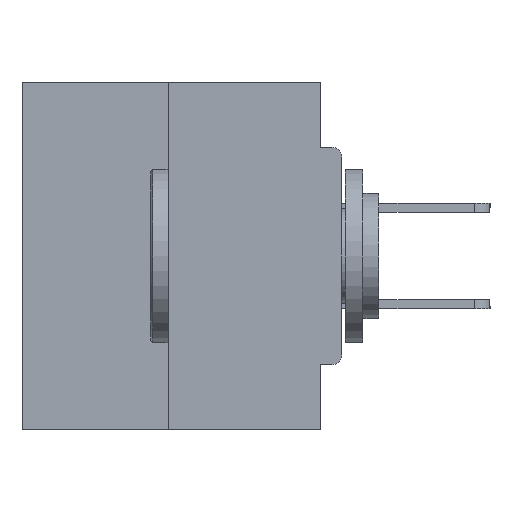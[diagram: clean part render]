
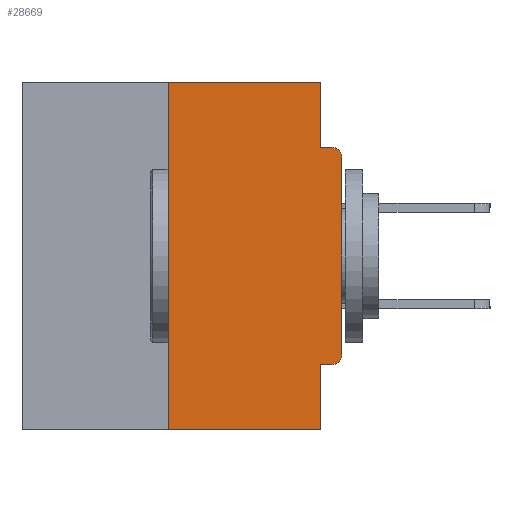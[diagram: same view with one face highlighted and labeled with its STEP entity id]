
A CAD part, left-side view. The second image highlights one B-rep face of the part: STEP entity #28669.
In plain terms, the highlighted planar face has unit normal (-1, 0, 0).
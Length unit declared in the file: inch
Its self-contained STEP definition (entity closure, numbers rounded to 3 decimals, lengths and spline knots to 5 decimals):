
#170 = AXIS2_PLACEMENT_3D ( 'NONE', #29297, #12699, #24218 ) ;
#797 = CIRCLE ( 'NONE', #20504, 0.015 ) ;
#966 = CARTESIAN_POINT ( 'NONE',  ( 0., 0.46, 0. ) ) ;
#1132 = VERTEX_POINT ( 'NONE', #33393 ) ;
#2004 = VERTEX_POINT ( 'NONE', #34199 ) ;
#2018 = CARTESIAN_POINT ( 'NONE',  ( 0., 0., 0. ) ) ;
#2049 = CARTESIAN_POINT ( 'NONE',  ( 0., 0.015, -0.0935 ) ) ;
#2283 = VECTOR ( 'NONE', #7430, 39.37008 ) ;
#2416 = DIRECTION ( 'NONE',  ( 0., 0., -1. ) ) ;
#3641 = ORIENTED_EDGE ( 'NONE', *, *, #21033, .T. ) ;
#3887 = ORIENTED_EDGE ( 'NONE', *, *, #13370, .F. ) ;
#4322 = CARTESIAN_POINT ( 'NONE',  ( 0., 0., -0.0935 ) ) ;
#4519 = CARTESIAN_POINT ( 'NONE',  ( 0., 0.25, -0.5 ) ) ;
#6406 = CARTESIAN_POINT ( 'NONE',  ( 0., 0.25, 0. ) ) ;
#6606 = LINE ( 'NONE', #4322, #2283 ) ;
#7320 = ORIENTED_EDGE ( 'NONE', *, *, #13843, .F. ) ;
#7430 = DIRECTION ( 'NONE',  ( 0., -1., 0. ) ) ;
#7748 = VERTEX_POINT ( 'NONE', #35030 ) ;
#8497 = EDGE_CURVE ( 'NONE', #1132, #11065, #6606, .T. ) ;
#8674 = ORIENTED_EDGE ( 'NONE', *, *, #22749, .T. ) ;
#8879 = VECTOR ( 'NONE', #33861, 39.37008 ) ;
#9446 = VECTOR ( 'NONE', #20384, 39.37008 ) ;
#9640 = CARTESIAN_POINT ( 'NONE',  ( 0., 0., -0.1085 ) ) ;
#9880 = EDGE_CURVE ( 'NONE', #20955, #14867, #30779, .T. ) ;
#10159 = CARTESIAN_POINT ( 'NONE',  ( 0., 0.015, -0.3915 ) ) ;
#10574 = CARTESIAN_POINT ( 'NONE',  ( 0., 0.015, -0.4065 ) ) ;
#10681 = CARTESIAN_POINT ( 'NONE',  ( 0., 0.46, -0.5 ) ) ;
#11065 = VERTEX_POINT ( 'NONE', #2049 ) ;
#12275 = EDGE_CURVE ( 'NONE', #13109, #32064, #32532, .T. ) ;
#12554 = LINE ( 'NONE', #6406, #8879 ) ;
#12572 = PLANE ( 'NONE',  #170 ) ;
#12699 = DIRECTION ( 'NONE',  ( 1., 0., 0. ) ) ;
#12783 = AXIS2_PLACEMENT_3D ( 'NONE', #21196, #20721, #34601 ) ;
#12846 = DIRECTION ( 'NONE',  ( -1., 0., 0. ) ) ;
#13091 = LINE ( 'NONE', #2018, #30837 ) ;
#13109 = VERTEX_POINT ( 'NONE', #4519 ) ;
#13370 = EDGE_CURVE ( 'NONE', #13109, #7748, #12554, .T. ) ;
#13621 = EDGE_CURVE ( 'NONE', #17387, #1132, #32442, .T. ) ;
#13722 = CARTESIAN_POINT ( 'NONE',  ( 0., 0.031, 0. ) ) ;
#13843 = EDGE_CURVE ( 'NONE', #7748, #17387, #17719, .T. ) ;
#14002 = EDGE_CURVE ( 'NONE', #20955, #2004, #797, .T. ) ;
#14108 = CARTESIAN_POINT ( 'NONE',  ( 0., 0.031, -0.5 ) ) ;
#14200 = EDGE_CURVE ( 'NONE', #14867, #32064, #22891, .T. ) ;
#14867 = VERTEX_POINT ( 'NONE', #21730 ) ;
#14953 = CARTESIAN_POINT ( 'NONE',  ( 0., 0.031, 0. ) ) ;
#16198 = FACE_OUTER_BOUND ( 'NONE', #16829, .T. ) ;
#16272 = DIRECTION ( 'NONE',  ( 0., -1., 0. ) ) ;
#16620 = DIRECTION ( 'NONE',  ( 0., 0., -1. ) ) ;
#16829 = EDGE_LOOP ( 'NONE', ( #7320, #3887, #19017, #27367, #26257, #17218, #3641, #8674, #25823, #29649 ) ) ;
#17218 = ORIENTED_EDGE ( 'NONE', *, *, #14002, .T. ) ;
#17387 = VERTEX_POINT ( 'NONE', #14953 ) ;
#17719 = LINE ( 'NONE', #966, #9446 ) ;
#17740 = CARTESIAN_POINT ( 'NONE',  ( 0., 0., -0.4065 ) ) ;
#18272 = VECTOR ( 'NONE', #16272, 39.37008 ) ;
#19017 = ORIENTED_EDGE ( 'NONE', *, *, #12275, .T. ) ;
#19019 = CARTESIAN_POINT ( 'NONE',  ( 0., 0.031, -0.5 ) ) ;
#20384 = DIRECTION ( 'NONE',  ( 0., -1., 0. ) ) ;
#20504 = AXIS2_PLACEMENT_3D ( 'NONE', #10159, #12846, #29456 ) ;
#20721 = DIRECTION ( 'NONE',  ( -1., 0., 0. ) ) ;
#20955 = VERTEX_POINT ( 'NONE', #10574 ) ;
#21033 = EDGE_CURVE ( 'NONE', #2004, #35524, #13091, .T. ) ;
#21196 = CARTESIAN_POINT ( 'NONE',  ( 0., 0.015, -0.1085 ) ) ;
#21730 = CARTESIAN_POINT ( 'NONE',  ( 0., 0.031, -0.4065 ) ) ;
#22749 = EDGE_CURVE ( 'NONE', #35524, #11065, #30717, .T. ) ;
#22891 = LINE ( 'NONE', #19019, #24640 ) ;
#24218 = DIRECTION ( 'NONE',  ( 0., 0., -1. ) ) ;
#24640 = VECTOR ( 'NONE', #2416, 39.37008 ) ;
#25823 = ORIENTED_EDGE ( 'NONE', *, *, #8497, .F. ) ;
#26231 = DIRECTION ( 'NONE',  ( 0., 1., 0. ) ) ;
#26257 = ORIENTED_EDGE ( 'NONE', *, *, #9880, .F. ) ;
#27367 = ORIENTED_EDGE ( 'NONE', *, *, #14200, .F. ) ;
#28669 = ADVANCED_FACE ( 'NONE', ( #16198 ), #12572, .F. ) ;
#29297 = CARTESIAN_POINT ( 'NONE',  ( 0., 0.46, 0. ) ) ;
#29456 = DIRECTION ( 'NONE',  ( 0., 0., -1. ) ) ;
#29649 = ORIENTED_EDGE ( 'NONE', *, *, #13621, .F. ) ;
#29762 = DIRECTION ( 'NONE',  ( 0., 0., 1. ) ) ;
#30379 = VECTOR ( 'NONE', #26231, 39.37008 ) ;
#30717 = CIRCLE ( 'NONE', #12783, 0.015 ) ;
#30779 = LINE ( 'NONE', #17740, #30379 ) ;
#30837 = VECTOR ( 'NONE', #29762, 39.37008 ) ;
#32003 = VECTOR ( 'NONE', #16620, 39.37008 ) ;
#32064 = VERTEX_POINT ( 'NONE', #14108 ) ;
#32442 = LINE ( 'NONE', #13722, #32003 ) ;
#32532 = LINE ( 'NONE', #10681, #18272 ) ;
#33393 = CARTESIAN_POINT ( 'NONE',  ( 0., 0.031, -0.0935 ) ) ;
#33861 = DIRECTION ( 'NONE',  ( 0., 0., 1. ) ) ;
#34199 = CARTESIAN_POINT ( 'NONE',  ( 0., 0., -0.3915 ) ) ;
#34601 = DIRECTION ( 'NONE',  ( 0., 0., -1. ) ) ;
#35030 = CARTESIAN_POINT ( 'NONE',  ( 0., 0.25, 0. ) ) ;
#35524 = VERTEX_POINT ( 'NONE', #9640 ) ;
